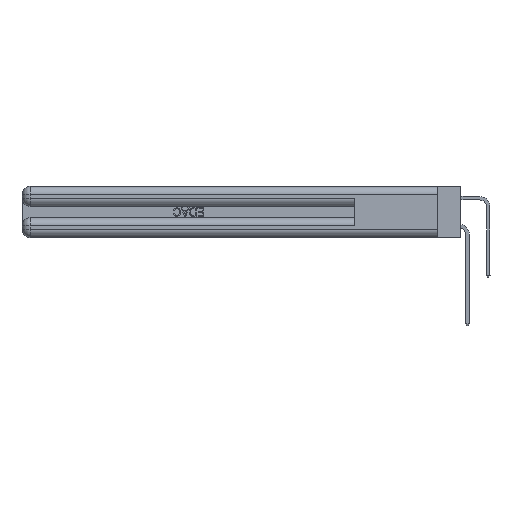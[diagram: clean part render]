
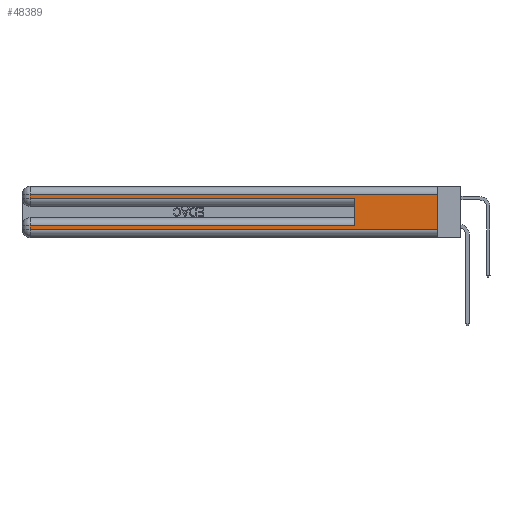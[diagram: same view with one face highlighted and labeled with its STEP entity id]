
A CAD part, left-side view. The second image highlights one B-rep face of the part: STEP entity #48389.
In plain terms, the highlighted planar face has unit normal (-1, 0, 0).
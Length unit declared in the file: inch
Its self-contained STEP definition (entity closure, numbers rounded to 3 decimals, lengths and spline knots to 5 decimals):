
#92 = ORIENTED_EDGE ( 'NONE', *, *, #16105, .T. ) ;
#314 = VECTOR ( 'NONE', #8628, 39.37008 ) ;
#2783 = ORIENTED_EDGE ( 'NONE', *, *, #30460, .F. ) ;
#3002 = EDGE_LOOP ( 'NONE', ( #24822, #9131, #37973, #24331, #2783, #92, #12058, #43958 ) ) ;
#3900 = VERTEX_POINT ( 'NONE', #44950 ) ;
#4339 = VECTOR ( 'NONE', #22396, 39.37008 ) ;
#4746 = VECTOR ( 'NONE', #35012, 39.37008 ) ;
#5461 = DIRECTION ( 'NONE',  ( 0., 1., 0. ) ) ;
#5973 = VECTOR ( 'NONE', #36054, 39.37008 ) ;
#6260 = EDGE_CURVE ( 'NONE', #29876, #3900, #39850, .T. ) ;
#7256 = CARTESIAN_POINT ( 'NONE',  ( 0., 0., 0.06 ) ) ;
#7319 = VERTEX_POINT ( 'NONE', #46498 ) ;
#7652 = CARTESIAN_POINT ( 'NONE',  ( 0., 0.6, 0.085 ) ) ;
#8628 = DIRECTION ( 'NONE',  ( 0., -1., 0. ) ) ;
#9131 = ORIENTED_EDGE ( 'NONE', *, *, #39191, .T. ) ;
#10386 = CARTESIAN_POINT ( 'NONE',  ( 0., 0., 0.085 ) ) ;
#10490 = LINE ( 'NONE', #30960, #314 ) ;
#12058 = ORIENTED_EDGE ( 'NONE', *, *, #17085, .T. ) ;
#12417 = LINE ( 'NONE', #16649, #5973 ) ;
#12541 = LINE ( 'NONE', #34886, #39091 ) ;
#12978 = EDGE_CURVE ( 'NONE', #7319, #25697, #12417, .T. ) ;
#14896 = VERTEX_POINT ( 'NONE', #28232 ) ;
#16105 = EDGE_CURVE ( 'NONE', #44643, #47668, #42233, .T. ) ;
#16262 = VECTOR ( 'NONE', #5461, 39.37008 ) ;
#16649 = CARTESIAN_POINT ( 'NONE',  ( 0., 2.94, 0.37 ) ) ;
#16904 = DIRECTION ( 'NONE',  ( 0., 0., -1. ) ) ;
#17085 = EDGE_CURVE ( 'NONE', #47668, #29876, #17885, .T. ) ;
#17885 = LINE ( 'NONE', #31833, #40975 ) ;
#19000 = AXIS2_PLACEMENT_3D ( 'NONE', #47312, #46963, #42283 ) ;
#19142 = VECTOR ( 'NONE', #23322, 39.37008 ) ;
#21739 = VERTEX_POINT ( 'NONE', #42817 ) ;
#22396 = DIRECTION ( 'NONE',  ( 0., -1., 0. ) ) ;
#22958 = CARTESIAN_POINT ( 'NONE',  ( 0., 2.94, 0.285 ) ) ;
#23322 = DIRECTION ( 'NONE',  ( 0., 1., 0. ) ) ;
#24331 = ORIENTED_EDGE ( 'NONE', *, *, #46471, .T. ) ;
#24383 = PLANE ( 'NONE',  #19000 ) ;
#24822 = ORIENTED_EDGE ( 'NONE', *, *, #31606, .F. ) ;
#25697 = VERTEX_POINT ( 'NONE', #22958 ) ;
#26909 = LINE ( 'NONE', #39331, #16262 ) ;
#28232 = CARTESIAN_POINT ( 'NONE',  ( 0., 0., 0.31 ) ) ;
#29876 = VERTEX_POINT ( 'NONE', #46823 ) ;
#30208 = LINE ( 'NONE', #31387, #4746 ) ;
#30460 = EDGE_CURVE ( 'NONE', #44643, #21739, #30208, .T. ) ;
#30960 = CARTESIAN_POINT ( 'NONE',  ( 0., 0., 0.285 ) ) ;
#31387 = CARTESIAN_POINT ( 'NONE',  ( 0., 0.6, 0.145 ) ) ;
#31606 = EDGE_CURVE ( 'NONE', #14896, #3900, #12541, .T. ) ;
#31617 = FACE_OUTER_BOUND ( 'NONE', #3002, .T. ) ;
#31833 = CARTESIAN_POINT ( 'NONE',  ( 0., 2.94, 0.37 ) ) ;
#34886 = CARTESIAN_POINT ( 'NONE',  ( 0., 0., 0.37 ) ) ;
#35012 = DIRECTION ( 'NONE',  ( 0., 0., 1. ) ) ;
#36054 = DIRECTION ( 'NONE',  ( 0., 0., -1. ) ) ;
#37973 = ORIENTED_EDGE ( 'NONE', *, *, #12978, .T. ) ;
#38991 = DIRECTION ( 'NONE',  ( 0., 0., -1. ) ) ;
#39091 = VECTOR ( 'NONE', #38991, 39.37008 ) ;
#39191 = EDGE_CURVE ( 'NONE', #14896, #7319, #26909, .T. ) ;
#39331 = CARTESIAN_POINT ( 'NONE',  ( 0., 0., 0.31 ) ) ;
#39850 = LINE ( 'NONE', #7256, #4339 ) ;
#40975 = VECTOR ( 'NONE', #16904, 39.37008 ) ;
#41218 = CARTESIAN_POINT ( 'NONE',  ( 0., 2.94, 0.085 ) ) ;
#42233 = LINE ( 'NONE', #10386, #19142 ) ;
#42283 = DIRECTION ( 'NONE',  ( 0., 0., -1. ) ) ;
#42817 = CARTESIAN_POINT ( 'NONE',  ( 0., 0.6, 0.285 ) ) ;
#43958 = ORIENTED_EDGE ( 'NONE', *, *, #6260, .T. ) ;
#44643 = VERTEX_POINT ( 'NONE', #7652 ) ;
#44950 = CARTESIAN_POINT ( 'NONE',  ( 0., 0., 0.06 ) ) ;
#46471 = EDGE_CURVE ( 'NONE', #25697, #21739, #10490, .T. ) ;
#46498 = CARTESIAN_POINT ( 'NONE',  ( 0., 2.94, 0.31 ) ) ;
#46823 = CARTESIAN_POINT ( 'NONE',  ( 0., 2.94, 0.06 ) ) ;
#46963 = DIRECTION ( 'NONE',  ( 1., 0., 0. ) ) ;
#47312 = CARTESIAN_POINT ( 'NONE',  ( 0., 0., 0.37 ) ) ;
#47668 = VERTEX_POINT ( 'NONE', #41218 ) ;
#48389 = ADVANCED_FACE ( 'NONE', ( #31617 ), #24383, .F. ) ;
